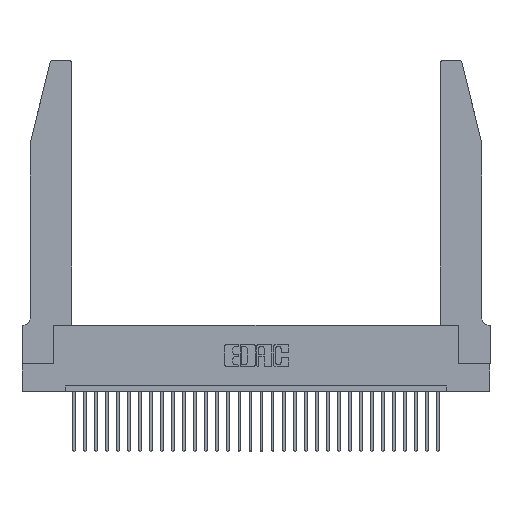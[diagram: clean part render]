
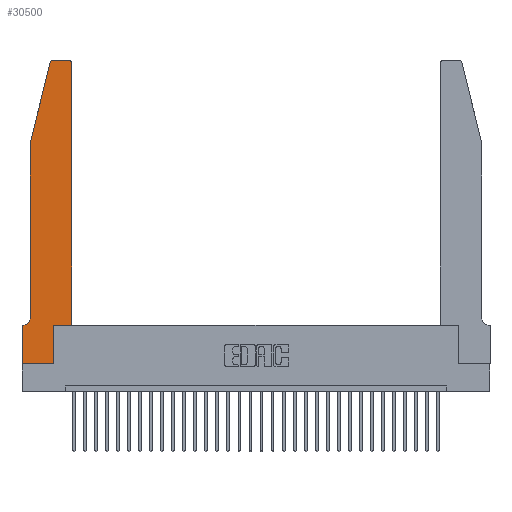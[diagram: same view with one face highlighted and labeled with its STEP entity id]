
A CAD part, top view. The second image highlights one B-rep face of the part: STEP entity #30500.
In plain terms, the highlighted planar face has unit normal (0, 0, 1).
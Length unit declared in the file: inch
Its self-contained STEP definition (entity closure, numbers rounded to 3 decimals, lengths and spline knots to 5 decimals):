
#148 = EDGE_CURVE ( 'NONE', #24784, #10092, #793, .T. ) ;
#322 = VECTOR ( 'NONE', #7578, 39.37008 ) ;
#471 = DIRECTION ( 'NONE',  ( -1., 0., 0. ) ) ;
#793 = CIRCLE ( 'NONE', #15289, 0.03 ) ;
#952 = ORIENTED_EDGE ( 'NONE', *, *, #19533, .T. ) ;
#1074 = DIRECTION ( 'NONE',  ( 0., 0., 1. ) ) ;
#1955 = ORIENTED_EDGE ( 'NONE', *, *, #3716, .T. ) ;
#1956 = DIRECTION ( 'NONE',  ( -1., 0., 0. ) ) ;
#2580 = EDGE_CURVE ( 'NONE', #3113, #11017, #22582, .T. ) ;
#2954 = ORIENTED_EDGE ( 'NONE', *, *, #8734, .T. ) ;
#2978 = DIRECTION ( 'NONE',  ( 1., 0., 0. ) ) ;
#3047 = EDGE_CURVE ( 'NONE', #10375, #15442, #31332, .T. ) ;
#3113 = VERTEX_POINT ( 'NONE', #25177 ) ;
#3124 = LINE ( 'NONE', #27560, #14482 ) ;
#3173 = CARTESIAN_POINT ( 'NONE',  ( 0.284, 2.72, 0.37 ) ) ;
#3178 = VECTOR ( 'NONE', #6313, 39.37008 ) ;
#3716 = EDGE_CURVE ( 'NONE', #10092, #3113, #23278, .T. ) ;
#3974 = CARTESIAN_POINT ( 'NONE',  ( 0., 0., 0.37 ) ) ;
#4110 = CARTESIAN_POINT ( 'NONE',  ( 0.4505, 0.35, 0.37 ) ) ;
#4258 = ORIENTED_EDGE ( 'NONE', *, *, #18669, .T. ) ;
#4516 = EDGE_CURVE ( 'NONE', #9223, #6103, #3124, .T. ) ;
#4637 = DIRECTION ( 'NONE',  ( 0., 0., 1. ) ) ;
#5070 = EDGE_CURVE ( 'NONE', #11017, #27475, #30925, .T. ) ;
#5385 = ORIENTED_EDGE ( 'NONE', *, *, #4516, .T. ) ;
#5392 = ORIENTED_EDGE ( 'NONE', *, *, #2580, .T. ) ;
#5932 = DIRECTION ( 'NONE',  ( 1., 0., 0. ) ) ;
#6103 = VERTEX_POINT ( 'NONE', #9184 ) ;
#6198 = CARTESIAN_POINT ( 'NONE',  ( 0.2605, 2.75, 0.37 ) ) ;
#6246 = PLANE ( 'NONE',  #16654 ) ;
#6313 = DIRECTION ( 'NONE',  ( -1., 0., 0. ) ) ;
#6336 = VECTOR ( 'NONE', #18764, 39.37008 ) ;
#6415 = DIRECTION ( 'NONE',  ( 1., 0., 0. ) ) ;
#7027 = EDGE_LOOP ( 'NONE', ( #1955, #5392, #14848, #2954, #4258, #11385, #15220, #25894, #5385, #952, #29113, #8295 ) ) ;
#7427 = CARTESIAN_POINT ( 'NONE',  ( 0.4505, 0.35, 0.37 ) ) ;
#7578 = DIRECTION ( 'NONE',  ( 1., 0., 0. ) ) ;
#7856 = LINE ( 'NONE', #19864, #322 ) ;
#8079 = CARTESIAN_POINT ( 'NONE',  ( 0.2865, 0., 0.37 ) ) ;
#8295 = ORIENTED_EDGE ( 'NONE', *, *, #148, .T. ) ;
#8734 = EDGE_CURVE ( 'NONE', #27475, #21478, #27984, .T. ) ;
#9009 = CIRCLE ( 'NONE', #16687, 0.07 ) ;
#9184 = CARTESIAN_POINT ( 'NONE',  ( 0.2865, 0.35, 0.37 ) ) ;
#9223 = VERTEX_POINT ( 'NONE', #8079 ) ;
#10092 = VERTEX_POINT ( 'NONE', #26513 ) ;
#10375 = VERTEX_POINT ( 'NONE', #12995 ) ;
#11017 = VERTEX_POINT ( 'NONE', #27368 ) ;
#11211 = VERTEX_POINT ( 'NONE', #24453 ) ;
#11345 = AXIS2_PLACEMENT_3D ( 'NONE', #3173, #24706, #2978 ) ;
#11385 = ORIENTED_EDGE ( 'NONE', *, *, #20869, .T. ) ;
#12172 = CARTESIAN_POINT ( 'NONE',  ( 0.4505, 2.72, 0.37 ) ) ;
#12537 = LINE ( 'NONE', #3974, #24332 ) ;
#12816 = LINE ( 'NONE', #4110, #28390 ) ;
#12995 = CARTESIAN_POINT ( 'NONE',  ( 0., 0.35, 0.37 ) ) ;
#13081 = VECTOR ( 'NONE', #17424, 39.37008 ) ;
#13233 = CARTESIAN_POINT ( 'NONE',  ( 0.0755, 0.42, 0.37 ) ) ;
#14108 = VERTEX_POINT ( 'NONE', #7427 ) ;
#14482 = VECTOR ( 'NONE', #15009, 39.37008 ) ;
#14848 = ORIENTED_EDGE ( 'NONE', *, *, #5070, .T. ) ;
#14851 = CARTESIAN_POINT ( 'NONE',  ( 0., 0., 0.37 ) ) ;
#15009 = DIRECTION ( 'NONE',  ( 0., 1., 0. ) ) ;
#15088 = DIRECTION ( 'NONE',  ( -0.239, -0.971, 0. ) ) ;
#15129 = VECTOR ( 'NONE', #471, 39.37008 ) ;
#15220 = ORIENTED_EDGE ( 'NONE', *, *, #3047, .T. ) ;
#15289 = AXIS2_PLACEMENT_3D ( 'NONE', #24139, #4637, #26595 ) ;
#15442 = VERTEX_POINT ( 'NONE', #14851 ) ;
#16654 = AXIS2_PLACEMENT_3D ( 'NONE', #20798, #1074, #5932 ) ;
#16687 = AXIS2_PLACEMENT_3D ( 'NONE', #24019, #26265, #1956 ) ;
#16828 = EDGE_CURVE ( 'NONE', #15442, #9223, #12537, .T. ) ;
#17082 = CARTESIAN_POINT ( 'NONE',  ( 0.0755, 0.35, 0.37 ) ) ;
#17424 = DIRECTION ( 'NONE',  ( 0., -1., 0. ) ) ;
#17630 = CARTESIAN_POINT ( 'NONE',  ( 0., 0., 0.37 ) ) ;
#18336 = VECTOR ( 'NONE', #15088, 39.37008 ) ;
#18669 = EDGE_CURVE ( 'NONE', #21478, #11211, #9009, .T. ) ;
#18764 = DIRECTION ( 'NONE',  ( 0., -1., 0. ) ) ;
#19334 = EDGE_CURVE ( 'NONE', #14108, #24784, #12816, .T. ) ;
#19533 = EDGE_CURVE ( 'NONE', #6103, #14108, #7856, .T. ) ;
#19864 = CARTESIAN_POINT ( 'NONE',  ( 0.4505, 0.35, 0.37 ) ) ;
#20798 = CARTESIAN_POINT ( 'NONE',  ( 0., 0.35, 0.37 ) ) ;
#20869 = EDGE_CURVE ( 'NONE', #11211, #10375, #21639, .T. ) ;
#21478 = VERTEX_POINT ( 'NONE', #13233 ) ;
#21639 = LINE ( 'NONE', #17082, #15129 ) ;
#22582 = CIRCLE ( 'NONE', #11345, 0.03 ) ;
#22641 = FACE_OUTER_BOUND ( 'NONE', #7027, .T. ) ;
#23278 = LINE ( 'NONE', #6198, #3178 ) ;
#24019 = CARTESIAN_POINT ( 'NONE',  ( 0.0055, 0.42, 0.37 ) ) ;
#24139 = CARTESIAN_POINT ( 'NONE',  ( 0.4205, 2.72, 0.37 ) ) ;
#24332 = VECTOR ( 'NONE', #6415, 39.37008 ) ;
#24453 = CARTESIAN_POINT ( 'NONE',  ( 0.0055, 0.35, 0.37 ) ) ;
#24706 = DIRECTION ( 'NONE',  ( 0., 0., 1. ) ) ;
#24784 = VERTEX_POINT ( 'NONE', #12172 ) ;
#25177 = CARTESIAN_POINT ( 'NONE',  ( 0.284, 2.75, 0.37 ) ) ;
#25894 = ORIENTED_EDGE ( 'NONE', *, *, #16828, .T. ) ;
#26265 = DIRECTION ( 'NONE',  ( 0., 0., -1. ) ) ;
#26513 = CARTESIAN_POINT ( 'NONE',  ( 0.4205, 2.75, 0.37 ) ) ;
#26595 = DIRECTION ( 'NONE',  ( 1., 0., 0. ) ) ;
#27368 = CARTESIAN_POINT ( 'NONE',  ( 0.25487, 2.72718, 0.37 ) ) ;
#27442 = CARTESIAN_POINT ( 'NONE',  ( 0.0755, 2., 0.37 ) ) ;
#27475 = VERTEX_POINT ( 'NONE', #27442 ) ;
#27560 = CARTESIAN_POINT ( 'NONE',  ( 0.2865, 0.35, 0.37 ) ) ;
#27984 = LINE ( 'NONE', #30993, #6336 ) ;
#28390 = VECTOR ( 'NONE', #30955, 39.37008 ) ;
#29113 = ORIENTED_EDGE ( 'NONE', *, *, #19334, .T. ) ;
#29669 = CARTESIAN_POINT ( 'NONE',  ( 0.0755, 2., 0.37 ) ) ;
#30500 = ADVANCED_FACE ( 'NONE', ( #22641 ), #6246, .T. ) ;
#30925 = LINE ( 'NONE', #29669, #18336 ) ;
#30955 = DIRECTION ( 'NONE',  ( 0., 1., 0. ) ) ;
#30993 = CARTESIAN_POINT ( 'NONE',  ( 0.0755, 2., 0.37 ) ) ;
#31332 = LINE ( 'NONE', #17630, #13081 ) ;
